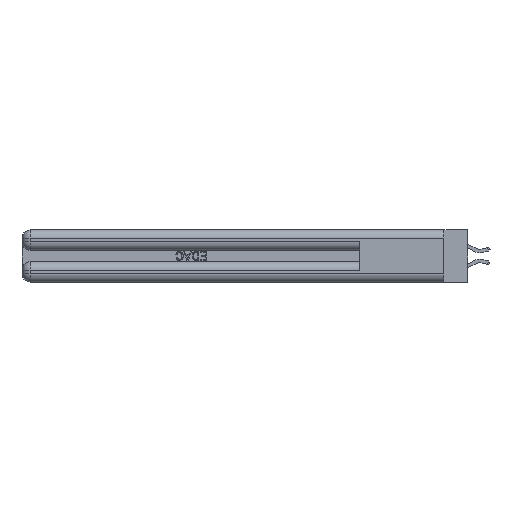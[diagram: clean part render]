
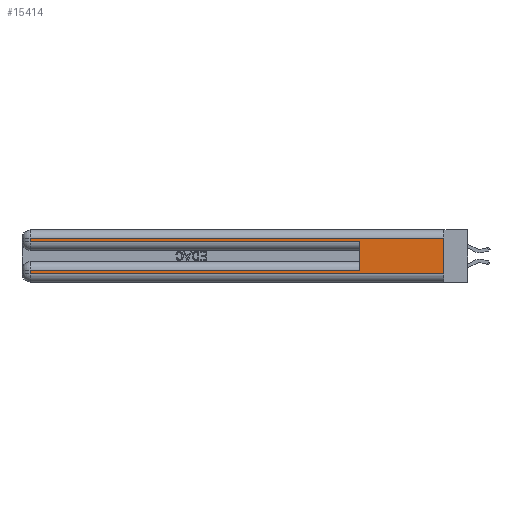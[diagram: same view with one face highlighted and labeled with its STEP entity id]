
A CAD part, left-side view. The second image highlights one B-rep face of the part: STEP entity #15414.
In plain terms, the highlighted planar face has unit normal (-1, 0, 0).
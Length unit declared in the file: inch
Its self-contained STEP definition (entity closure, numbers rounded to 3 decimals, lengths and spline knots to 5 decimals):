
#408 = DIRECTION ( 'NONE',  ( 0., -1., 0. ) ) ;
#441 = ORIENTED_EDGE ( 'NONE', *, *, #33213, .T. ) ;
#599 = CARTESIAN_POINT ( 'NONE',  ( 0., 0., 0.085 ) ) ;
#1292 = CARTESIAN_POINT ( 'NONE',  ( 0., 0., 0.37 ) ) ;
#1481 = CARTESIAN_POINT ( 'NONE',  ( 0., 0., 0.06 ) ) ;
#2549 = VERTEX_POINT ( 'NONE', #32929 ) ;
#4250 = CARTESIAN_POINT ( 'NONE',  ( 0., 0.6, 0.145 ) ) ;
#4415 = VECTOR ( 'NONE', #23678, 39.37008 ) ;
#4909 = LINE ( 'NONE', #599, #18660 ) ;
#7370 = VECTOR ( 'NONE', #45075, 39.37008 ) ;
#7490 = LINE ( 'NONE', #15242, #13264 ) ;
#7731 = DIRECTION ( 'NONE',  ( 0., 0., -1. ) ) ;
#8123 = ORIENTED_EDGE ( 'NONE', *, *, #46576, .F. ) ;
#8498 = CARTESIAN_POINT ( 'NONE',  ( 0., 0.6, 0.085 ) ) ;
#8547 = DIRECTION ( 'NONE',  ( 0., 0., -1. ) ) ;
#8836 = EDGE_CURVE ( 'NONE', #42796, #30836, #7490, .T. ) ;
#9445 = CARTESIAN_POINT ( 'NONE',  ( 0., 2.94, 0.085 ) ) ;
#9506 = EDGE_CURVE ( 'NONE', #39175, #42796, #44326, .T. ) ;
#9958 = ORIENTED_EDGE ( 'NONE', *, *, #29047, .T. ) ;
#10556 = DIRECTION ( 'NONE',  ( 0., 0., -1. ) ) ;
#11881 = EDGE_CURVE ( 'NONE', #39175, #13607, #33955, .T. ) ;
#13264 = VECTOR ( 'NONE', #7731, 39.37008 ) ;
#13478 = CARTESIAN_POINT ( 'NONE',  ( 0., 2.94, 0.31 ) ) ;
#13607 = VERTEX_POINT ( 'NONE', #46756 ) ;
#14789 = EDGE_CURVE ( 'NONE', #2549, #13607, #40085, .T. ) ;
#15242 = CARTESIAN_POINT ( 'NONE',  ( 0., 2.94, 0.37 ) ) ;
#15414 = ADVANCED_FACE ( 'NONE', ( #30870 ), #33922, .F. ) ;
#16112 = ORIENTED_EDGE ( 'NONE', *, *, #9506, .T. ) ;
#18283 = LINE ( 'NONE', #4250, #7370 ) ;
#18660 = VECTOR ( 'NONE', #44540, 39.37008 ) ;
#19777 = CARTESIAN_POINT ( 'NONE',  ( 0., 2.94, 0.285 ) ) ;
#19785 = LINE ( 'NONE', #23315, #28479 ) ;
#20247 = DIRECTION ( 'NONE',  ( 0., 1., 0. ) ) ;
#21367 = VERTEX_POINT ( 'NONE', #32935 ) ;
#22562 = CARTESIAN_POINT ( 'NONE',  ( 0., 0., 0.285 ) ) ;
#23155 = DIRECTION ( 'NONE',  ( 1., 0., 0. ) ) ;
#23315 = CARTESIAN_POINT ( 'NONE',  ( 0., 2.94, 0.37 ) ) ;
#23592 = ORIENTED_EDGE ( 'NONE', *, *, #14789, .T. ) ;
#23678 = DIRECTION ( 'NONE',  ( 0., -1., 0. ) ) ;
#24738 = ORIENTED_EDGE ( 'NONE', *, *, #44959, .T. ) ;
#26705 = DIRECTION ( 'NONE',  ( 0., 0., -1. ) ) ;
#27548 = AXIS2_PLACEMENT_3D ( 'NONE', #1292, #23155, #26705 ) ;
#27648 = CARTESIAN_POINT ( 'NONE',  ( 0., 0., 0.31 ) ) ;
#28479 = VECTOR ( 'NONE', #8547, 39.37008 ) ;
#29047 = EDGE_CURVE ( 'NONE', #32188, #2549, #19785, .T. ) ;
#29944 = LINE ( 'NONE', #22562, #37423 ) ;
#30836 = VERTEX_POINT ( 'NONE', #19777 ) ;
#30870 = FACE_OUTER_BOUND ( 'NONE', #46122, .T. ) ;
#32188 = VERTEX_POINT ( 'NONE', #9445 ) ;
#32230 = VECTOR ( 'NONE', #20247, 39.37008 ) ;
#32560 = CARTESIAN_POINT ( 'NONE',  ( 0., 0., 0.37 ) ) ;
#32929 = CARTESIAN_POINT ( 'NONE',  ( 0., 2.94, 0.06 ) ) ;
#32935 = CARTESIAN_POINT ( 'NONE',  ( 0., 0.6, 0.285 ) ) ;
#33213 = EDGE_CURVE ( 'NONE', #37006, #32188, #4909, .T. ) ;
#33922 = PLANE ( 'NONE',  #27548 ) ;
#33955 = LINE ( 'NONE', #32560, #43803 ) ;
#34883 = CARTESIAN_POINT ( 'NONE',  ( 0., 0., 0.31 ) ) ;
#36925 = ORIENTED_EDGE ( 'NONE', *, *, #11881, .F. ) ;
#37006 = VERTEX_POINT ( 'NONE', #8498 ) ;
#37423 = VECTOR ( 'NONE', #408, 39.37008 ) ;
#39175 = VERTEX_POINT ( 'NONE', #27648 ) ;
#39936 = ORIENTED_EDGE ( 'NONE', *, *, #8836, .T. ) ;
#40085 = LINE ( 'NONE', #1481, #4415 ) ;
#42796 = VERTEX_POINT ( 'NONE', #13478 ) ;
#43803 = VECTOR ( 'NONE', #10556, 39.37008 ) ;
#44326 = LINE ( 'NONE', #34883, #32230 ) ;
#44540 = DIRECTION ( 'NONE',  ( 0., 1., 0. ) ) ;
#44959 = EDGE_CURVE ( 'NONE', #30836, #21367, #29944, .T. ) ;
#45075 = DIRECTION ( 'NONE',  ( 0., 0., 1. ) ) ;
#46122 = EDGE_LOOP ( 'NONE', ( #36925, #16112, #39936, #24738, #8123, #441, #9958, #23592 ) ) ;
#46576 = EDGE_CURVE ( 'NONE', #37006, #21367, #18283, .T. ) ;
#46756 = CARTESIAN_POINT ( 'NONE',  ( 0., 0., 0.06 ) ) ;
